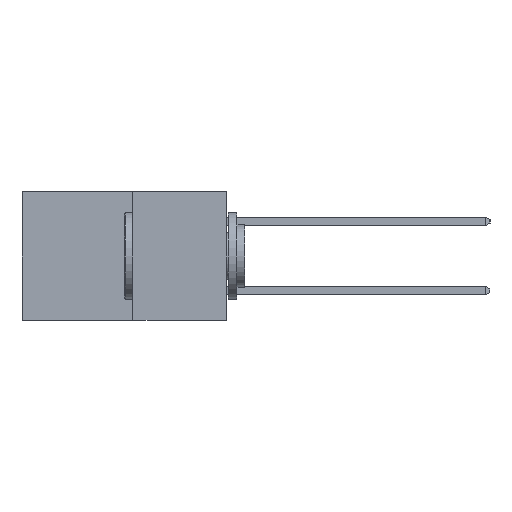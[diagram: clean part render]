
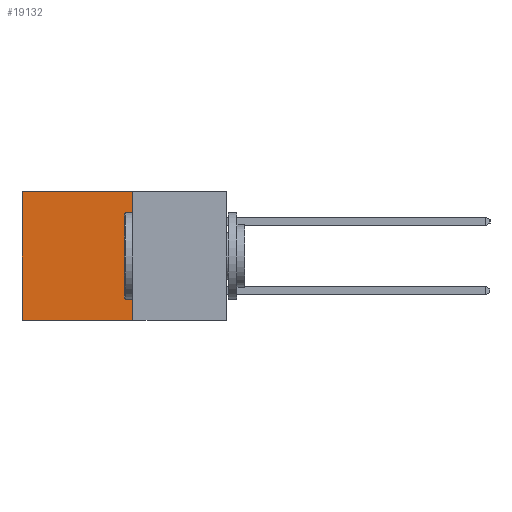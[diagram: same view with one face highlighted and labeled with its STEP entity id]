
A CAD part, left-side view. The second image highlights one B-rep face of the part: STEP entity #19132.
In plain terms, the highlighted planar face has unit normal (-1, 0, 0).
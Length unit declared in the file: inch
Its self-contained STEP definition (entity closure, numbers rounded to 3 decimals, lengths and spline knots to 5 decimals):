
#635 = CARTESIAN_POINT ( 'NONE',  ( 0.277, 0.59, 0. ) ) ;
#742 = PLANE ( 'NONE',  #5502 ) ;
#1956 = ORIENTED_EDGE ( 'NONE', *, *, #2834, .T. ) ;
#2516 = ORIENTED_EDGE ( 'NONE', *, *, #5527, .F. ) ;
#2834 = EDGE_CURVE ( 'NONE', #22238, #17442, #12501, .T. ) ;
#4588 = DIRECTION ( 'NONE',  ( 1., 0., 0. ) ) ;
#4797 = LINE ( 'NONE', #6143, #24186 ) ;
#4995 = VERTEX_POINT ( 'NONE', #12348 ) ;
#5004 = VECTOR ( 'NONE', #9095, 39.37008 ) ;
#5128 = EDGE_LOOP ( 'NONE', ( #1956, #2516, #7110, #11050 ) ) ;
#5502 = AXIS2_PLACEMENT_3D ( 'NONE', #14337, #4588, #18224 ) ;
#5527 = EDGE_CURVE ( 'NONE', #4995, #17442, #20516, .T. ) ;
#5799 = CARTESIAN_POINT ( 'NONE',  ( 0.277, 0.59, -0.37 ) ) ;
#6143 = CARTESIAN_POINT ( 'NONE',  ( 0.277, 0.27, -0.37 ) ) ;
#7110 = ORIENTED_EDGE ( 'NONE', *, *, #14951, .F. ) ;
#9091 = CARTESIAN_POINT ( 'NONE',  ( 0.277, 0.27, -0.37 ) ) ;
#9095 = DIRECTION ( 'NONE',  ( 0., 1., 0. ) ) ;
#9821 = VECTOR ( 'NONE', #16468, 39.37008 ) ;
#11050 = ORIENTED_EDGE ( 'NONE', *, *, #23049, .T. ) ;
#12348 = CARTESIAN_POINT ( 'NONE',  ( 0.277, 0.27, -0.37 ) ) ;
#12501 = LINE ( 'NONE', #17607, #22178 ) ;
#14337 = CARTESIAN_POINT ( 'NONE',  ( 0.277, 0.27, -0.37 ) ) ;
#14524 = CARTESIAN_POINT ( 'NONE',  ( 0.277, 0.27, 0. ) ) ;
#14951 = EDGE_CURVE ( 'NONE', #20764, #4995, #4797, .T. ) ;
#15979 = DIRECTION ( 'NONE',  ( 0., 0., -1. ) ) ;
#16468 = DIRECTION ( 'NONE',  ( 0., 1., 0. ) ) ;
#17320 = DIRECTION ( 'NONE',  ( 0., 0., -1. ) ) ;
#17442 = VERTEX_POINT ( 'NONE', #5799 ) ;
#17607 = CARTESIAN_POINT ( 'NONE',  ( 0.277, 0.59, -0.37 ) ) ;
#18224 = DIRECTION ( 'NONE',  ( 0., 0., -1. ) ) ;
#19132 = ADVANCED_FACE ( 'NONE', ( #21000 ), #742, .F. ) ;
#20137 = LINE ( 'NONE', #14524, #9821 ) ;
#20516 = LINE ( 'NONE', #9091, #5004 ) ;
#20764 = VERTEX_POINT ( 'NONE', #21779 ) ;
#21000 = FACE_OUTER_BOUND ( 'NONE', #5128, .T. ) ;
#21779 = CARTESIAN_POINT ( 'NONE',  ( 0.277, 0.27, 0. ) ) ;
#22178 = VECTOR ( 'NONE', #17320, 39.37008 ) ;
#22238 = VERTEX_POINT ( 'NONE', #635 ) ;
#23049 = EDGE_CURVE ( 'NONE', #20764, #22238, #20137, .T. ) ;
#24186 = VECTOR ( 'NONE', #15979, 39.37008 ) ;
